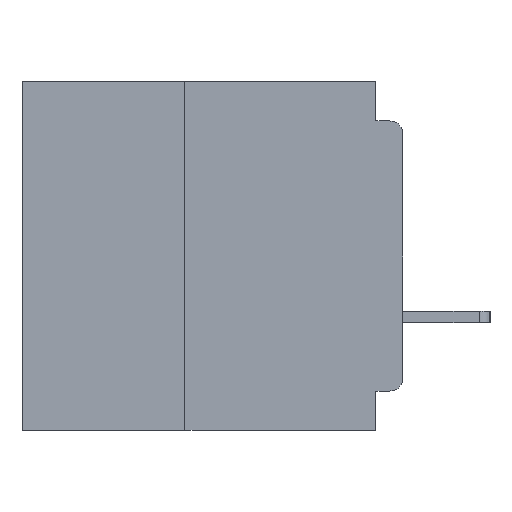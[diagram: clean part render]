
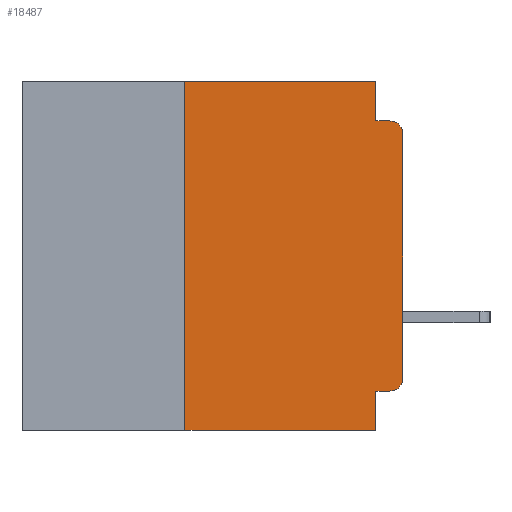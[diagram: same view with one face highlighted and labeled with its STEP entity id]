
A CAD part, left-side view. The second image highlights one B-rep face of the part: STEP entity #18487.
In plain terms, the highlighted planar face has unit normal (-1, 0, 0).
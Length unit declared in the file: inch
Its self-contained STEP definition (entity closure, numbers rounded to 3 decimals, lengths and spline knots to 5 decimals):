
#367 = CARTESIAN_POINT ( 'NONE',  ( 0., 0.437, 0. ) ) ;
#1582 = CARTESIAN_POINT ( 'NONE',  ( 0., 0.031, 0. ) ) ;
#1985 = CARTESIAN_POINT ( 'NONE',  ( 0., 0.031, -0.4 ) ) ;
#2473 = ORIENTED_EDGE ( 'NONE', *, *, #22816, .T. ) ;
#3157 = CARTESIAN_POINT ( 'NONE',  ( 0., 0., -0.06 ) ) ;
#3176 = VERTEX_POINT ( 'NONE', #29244 ) ;
#3402 = DIRECTION ( 'NONE',  ( 0., 0., -1. ) ) ;
#3893 = VERTEX_POINT ( 'NONE', #12752 ) ;
#5059 = VERTEX_POINT ( 'NONE', #26707 ) ;
#5698 = LINE ( 'NONE', #37288, #21704 ) ;
#5779 = ORIENTED_EDGE ( 'NONE', *, *, #10402, .F. ) ;
#6027 = LINE ( 'NONE', #1582, #22992 ) ;
#6127 = EDGE_CURVE ( 'NONE', #13196, #32315, #8036, .T. ) ;
#6322 = VECTOR ( 'NONE', #21981, 39.37008 ) ;
#7274 = CARTESIAN_POINT ( 'NONE',  ( 0., 0., -0.045 ) ) ;
#7523 = FACE_OUTER_BOUND ( 'NONE', #22287, .T. ) ;
#7798 = ORIENTED_EDGE ( 'NONE', *, *, #9821, .F. ) ;
#7880 = ORIENTED_EDGE ( 'NONE', *, *, #21079, .T. ) ;
#8036 = LINE ( 'NONE', #14335, #31156 ) ;
#8693 = CARTESIAN_POINT ( 'NONE',  ( 0., 0.015, -0.045 ) ) ;
#9279 = EDGE_CURVE ( 'NONE', #3893, #19479, #33244, .T. ) ;
#9821 = EDGE_CURVE ( 'NONE', #5059, #3176, #6027, .T. ) ;
#10402 = EDGE_CURVE ( 'NONE', #3176, #22848, #31429, .T. ) ;
#10606 = VERTEX_POINT ( 'NONE', #17138 ) ;
#10959 = DIRECTION ( 'NONE',  ( -1., 0., 0. ) ) ;
#11261 = VECTOR ( 'NONE', #35699, 39.37008 ) ;
#11414 = CIRCLE ( 'NONE', #15228, 0.015 ) ;
#11596 = CARTESIAN_POINT ( 'NONE',  ( 0., 0.437, -0.4 ) ) ;
#12226 = VECTOR ( 'NONE', #38490, 39.37008 ) ;
#12752 = CARTESIAN_POINT ( 'NONE',  ( 0., 0.015, -0.355 ) ) ;
#12896 = CARTESIAN_POINT ( 'NONE',  ( 0., 0.015, -0.06 ) ) ;
#12907 = CARTESIAN_POINT ( 'NONE',  ( 0., 0.031, -0.4 ) ) ;
#13196 = VERTEX_POINT ( 'NONE', #23053 ) ;
#14335 = CARTESIAN_POINT ( 'NONE',  ( 0., 0., 0. ) ) ;
#14358 = CARTESIAN_POINT ( 'NONE',  ( 0., 0.25, -0.4 ) ) ;
#14609 = ORIENTED_EDGE ( 'NONE', *, *, #6127, .T. ) ;
#15228 = AXIS2_PLACEMENT_3D ( 'NONE', #12896, #33963, #15908 ) ;
#15908 = DIRECTION ( 'NONE',  ( 0., 0., -1. ) ) ;
#16024 = VERTEX_POINT ( 'NONE', #23375 ) ;
#16355 = DIRECTION ( 'NONE',  ( 0., -1., 0. ) ) ;
#16433 = DIRECTION ( 'NONE',  ( 0., 1., 0. ) ) ;
#17138 = CARTESIAN_POINT ( 'NONE',  ( 0., 0.25, -0.4 ) ) ;
#18170 = VERTEX_POINT ( 'NONE', #1985 ) ;
#18330 = LINE ( 'NONE', #11596, #11261 ) ;
#18487 = ADVANCED_FACE ( 'NONE', ( #7523 ), #24333, .F. ) ;
#19209 = DIRECTION ( 'NONE',  ( 0., -1., 0. ) ) ;
#19479 = VERTEX_POINT ( 'NONE', #22761 ) ;
#21079 = EDGE_CURVE ( 'NONE', #32315, #22848, #11414, .T. ) ;
#21400 = DIRECTION ( 'NONE',  ( 1., 0., 0. ) ) ;
#21435 = CIRCLE ( 'NONE', #34280, 0.015 ) ;
#21704 = VECTOR ( 'NONE', #19209, 39.37008 ) ;
#21981 = DIRECTION ( 'NONE',  ( 0., 0., -1. ) ) ;
#22287 = EDGE_LOOP ( 'NONE', ( #14609, #7880, #5779, #7798, #30792, #27899, #2473, #29996, #24166, #33435 ) ) ;
#22595 = DIRECTION ( 'NONE',  ( 0., 0., -1. ) ) ;
#22755 = EDGE_CURVE ( 'NONE', #10606, #16024, #37216, .T. ) ;
#22761 = CARTESIAN_POINT ( 'NONE',  ( 0., 0.031, -0.355 ) ) ;
#22816 = EDGE_CURVE ( 'NONE', #10606, #18170, #18330, .T. ) ;
#22848 = VERTEX_POINT ( 'NONE', #8693 ) ;
#22992 = VECTOR ( 'NONE', #22595, 39.37008 ) ;
#23053 = CARTESIAN_POINT ( 'NONE',  ( 0., 0., -0.34 ) ) ;
#23375 = CARTESIAN_POINT ( 'NONE',  ( 0., 0.25, 0. ) ) ;
#24166 = ORIENTED_EDGE ( 'NONE', *, *, #9279, .F. ) ;
#24294 = VECTOR ( 'NONE', #16433, 39.37008 ) ;
#24333 = PLANE ( 'NONE',  #36892 ) ;
#25814 = EDGE_CURVE ( 'NONE', #3893, #13196, #21435, .T. ) ;
#26201 = EDGE_CURVE ( 'NONE', #19479, #18170, #38392, .T. ) ;
#26707 = CARTESIAN_POINT ( 'NONE',  ( 0., 0.031, 0. ) ) ;
#27899 = ORIENTED_EDGE ( 'NONE', *, *, #22755, .F. ) ;
#29015 = CARTESIAN_POINT ( 'NONE',  ( 0., 0.015, -0.34 ) ) ;
#29244 = CARTESIAN_POINT ( 'NONE',  ( 0., 0.031, -0.045 ) ) ;
#29996 = ORIENTED_EDGE ( 'NONE', *, *, #26201, .F. ) ;
#30792 = ORIENTED_EDGE ( 'NONE', *, *, #31908, .F. ) ;
#31156 = VECTOR ( 'NONE', #35418, 39.37008 ) ;
#31429 = LINE ( 'NONE', #7274, #38509 ) ;
#31461 = CARTESIAN_POINT ( 'NONE',  ( 0., 0., -0.355 ) ) ;
#31908 = EDGE_CURVE ( 'NONE', #16024, #5059, #5698, .T. ) ;
#32037 = DIRECTION ( 'NONE',  ( 0., 0., -1. ) ) ;
#32315 = VERTEX_POINT ( 'NONE', #3157 ) ;
#33244 = LINE ( 'NONE', #31461, #24294 ) ;
#33435 = ORIENTED_EDGE ( 'NONE', *, *, #25814, .T. ) ;
#33963 = DIRECTION ( 'NONE',  ( -1., 0., 0. ) ) ;
#34280 = AXIS2_PLACEMENT_3D ( 'NONE', #29015, #10959, #32037 ) ;
#35418 = DIRECTION ( 'NONE',  ( 0., 0., 1. ) ) ;
#35699 = DIRECTION ( 'NONE',  ( 0., -1., 0. ) ) ;
#36892 = AXIS2_PLACEMENT_3D ( 'NONE', #367, #21400, #3402 ) ;
#37216 = LINE ( 'NONE', #14358, #12226 ) ;
#37288 = CARTESIAN_POINT ( 'NONE',  ( 0., 0.437, 0. ) ) ;
#38392 = LINE ( 'NONE', #12907, #6322 ) ;
#38490 = DIRECTION ( 'NONE',  ( 0., 0., 1. ) ) ;
#38509 = VECTOR ( 'NONE', #16355, 39.37008 ) ;
